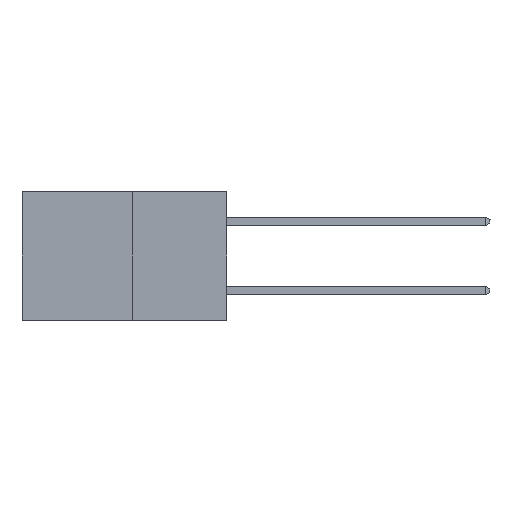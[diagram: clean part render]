
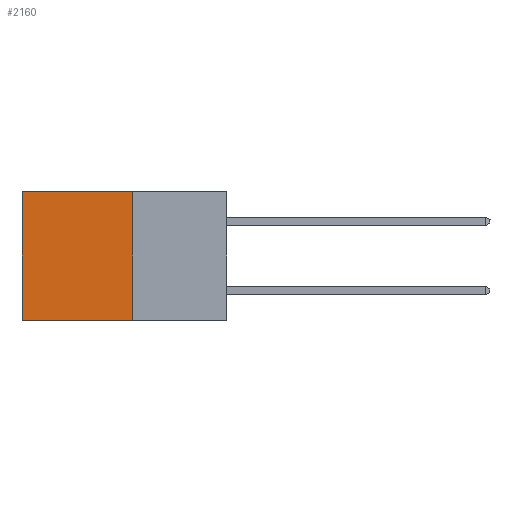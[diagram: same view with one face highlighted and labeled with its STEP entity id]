
A CAD part, left-side view. The second image highlights one B-rep face of the part: STEP entity #2160.
In plain terms, the highlighted planar face has unit normal (-1, 0, 0).
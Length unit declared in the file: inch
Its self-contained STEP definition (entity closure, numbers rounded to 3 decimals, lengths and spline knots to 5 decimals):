
#318 = EDGE_LOOP ( 'NONE', ( #13657, #13439, #6597, #1370 ) ) ;
#843 = FACE_OUTER_BOUND ( 'NONE', #318, .T. ) ;
#1318 = VERTEX_POINT ( 'NONE', #19697 ) ;
#1370 = ORIENTED_EDGE ( 'NONE', *, *, #7130, .T. ) ;
#1542 = DIRECTION ( 'NONE',  ( 0., 0., -1. ) ) ;
#1625 = VECTOR ( 'NONE', #10008, 39.37008 ) ;
#1695 = VECTOR ( 'NONE', #4908, 39.37008 ) ;
#1907 = EDGE_CURVE ( 'NONE', #15717, #4472, #6611, .T. ) ;
#2009 = CARTESIAN_POINT ( 'NONE',  ( 0.277, 0.27, 0. ) ) ;
#2160 = ADVANCED_FACE ( 'NONE', ( #843 ), #6915, .F. ) ;
#4472 = VERTEX_POINT ( 'NONE', #10793 ) ;
#4815 = VECTOR ( 'NONE', #9000, 39.37008 ) ;
#4908 = DIRECTION ( 'NONE',  ( 0., 1., 0. ) ) ;
#5516 = AXIS2_PLACEMENT_3D ( 'NONE', #6909, #13005, #1542 ) ;
#6597 = ORIENTED_EDGE ( 'NONE', *, *, #7376, .F. ) ;
#6611 = LINE ( 'NONE', #14706, #1625 ) ;
#6711 = DIRECTION ( 'NONE',  ( 0., 0., -1. ) ) ;
#6909 = CARTESIAN_POINT ( 'NONE',  ( 0.277, 0.27, -0.37 ) ) ;
#6915 = PLANE ( 'NONE',  #5516 ) ;
#7130 = EDGE_CURVE ( 'NONE', #9636, #15717, #12793, .T. ) ;
#7376 = EDGE_CURVE ( 'NONE', #9636, #1318, #9499, .T. ) ;
#8968 = CARTESIAN_POINT ( 'NONE',  ( 0.277, 0.27, 0. ) ) ;
#9000 = DIRECTION ( 'NONE',  ( 0., 1., 0. ) ) ;
#9050 = VECTOR ( 'NONE', #6711, 39.37008 ) ;
#9499 = LINE ( 'NONE', #12674, #9050 ) ;
#9636 = VERTEX_POINT ( 'NONE', #2009 ) ;
#10008 = DIRECTION ( 'NONE',  ( 0., 0., -1. ) ) ;
#10793 = CARTESIAN_POINT ( 'NONE',  ( 0.277, 0.59, -0.37 ) ) ;
#12129 = EDGE_CURVE ( 'NONE', #1318, #4472, #17300, .T. ) ;
#12674 = CARTESIAN_POINT ( 'NONE',  ( 0.277, 0.27, -0.37 ) ) ;
#12793 = LINE ( 'NONE', #8968, #4815 ) ;
#13005 = DIRECTION ( 'NONE',  ( 1., 0., 0. ) ) ;
#13439 = ORIENTED_EDGE ( 'NONE', *, *, #12129, .F. ) ;
#13657 = ORIENTED_EDGE ( 'NONE', *, *, #1907, .T. ) ;
#13802 = CARTESIAN_POINT ( 'NONE',  ( 0.277, 0.59, 0. ) ) ;
#14706 = CARTESIAN_POINT ( 'NONE',  ( 0.277, 0.59, -0.37 ) ) ;
#15401 = CARTESIAN_POINT ( 'NONE',  ( 0.277, 0.27, -0.37 ) ) ;
#15717 = VERTEX_POINT ( 'NONE', #13802 ) ;
#17300 = LINE ( 'NONE', #15401, #1695 ) ;
#19697 = CARTESIAN_POINT ( 'NONE',  ( 0.277, 0.27, -0.37 ) ) ;
